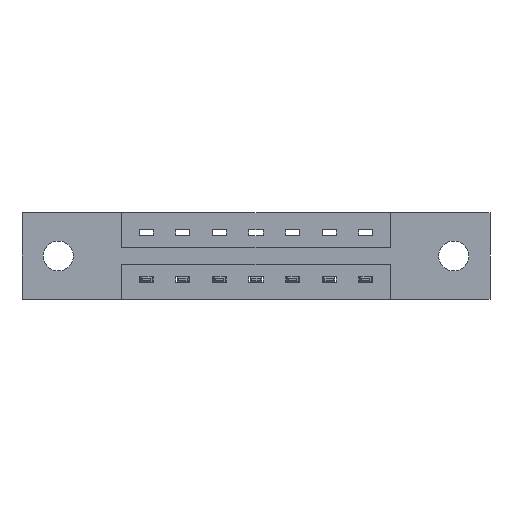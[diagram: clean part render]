
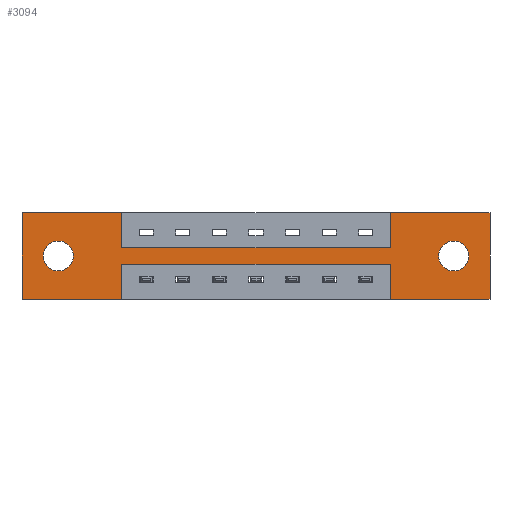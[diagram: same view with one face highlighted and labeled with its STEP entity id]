
A CAD part, front view. The second image highlights one B-rep face of the part: STEP entity #3094.
In plain terms, the highlighted planar face has unit normal (0, -1, 0).
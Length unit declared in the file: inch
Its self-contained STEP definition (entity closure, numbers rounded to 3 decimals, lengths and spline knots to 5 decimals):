
#146 = ORIENTED_EDGE ( 'NONE', *, *, #5167, .F. ) ;
#184 = ORIENTED_EDGE ( 'NONE', *, *, #8769, .F. ) ;
#269 = AXIS2_PLACEMENT_3D ( 'NONE', #9142, #9176, #1065 ) ;
#273 = VERTEX_POINT ( 'NONE', #4637 ) ;
#286 = CARTESIAN_POINT ( 'NONE',  ( 1.573, 0., -0.15 ) ) ;
#356 = CARTESIAN_POINT ( 'NONE',  ( 0.155, 0., -0.185 ) ) ;
#385 = LINE ( 'NONE', #4466, #8258 ) ;
#437 = CARTESIAN_POINT ( 'NONE',  ( 1.573, 0., -0.37 ) ) ;
#475 = VERTEX_POINT ( 'NONE', #6405 ) ;
#481 = ORIENTED_EDGE ( 'NONE', *, *, #5560, .F. ) ;
#738 = ORIENTED_EDGE ( 'NONE', *, *, #7618, .T. ) ;
#752 = LINE ( 'NONE', #7624, #9543 ) ;
#995 = DIRECTION ( 'NONE',  ( 0., 1., 0. ) ) ;
#1040 = VERTEX_POINT ( 'NONE', #6123 ) ;
#1065 = DIRECTION ( 'NONE',  ( 0., 0., 1. ) ) ;
#1081 = VERTEX_POINT ( 'NONE', #5333 ) ;
#1261 = CARTESIAN_POINT ( 'NONE',  ( 1.843, 0., -0.249 ) ) ;
#1365 = ORIENTED_EDGE ( 'NONE', *, *, #4331, .F. ) ;
#1369 = VECTOR ( 'NONE', #3549, 39.37008 ) ;
#1526 = EDGE_CURVE ( 'NONE', #7227, #5481, #5868, .T. ) ;
#1628 = LINE ( 'NONE', #2839, #7551 ) ;
#1788 = VECTOR ( 'NONE', #3250, 39.37008 ) ;
#1812 = EDGE_LOOP ( 'NONE', ( #8796, #6892 ) ) ;
#1844 = PLANE ( 'NONE',  #8091 ) ;
#1984 = VECTOR ( 'NONE', #8670, 39.37008 ) ;
#2133 = CARTESIAN_POINT ( 'NONE',  ( 1.573, 0., 0. ) ) ;
#2176 = DIRECTION ( 'NONE',  ( 0., -1., 0. ) ) ;
#2179 = CARTESIAN_POINT ( 'NONE',  ( 1.843, 0., -0.121 ) ) ;
#2238 = AXIS2_PLACEMENT_3D ( 'NONE', #7287, #5685, #8671 ) ;
#2365 = VECTOR ( 'NONE', #7357, 39.37008 ) ;
#2410 = FACE_OUTER_BOUND ( 'NONE', #8973, .T. ) ;
#2446 = CARTESIAN_POINT ( 'NONE',  ( 0., 0., 0. ) ) ;
#2516 = VERTEX_POINT ( 'NONE', #6598 ) ;
#2552 = CARTESIAN_POINT ( 'NONE',  ( 0.425, 0., -0.22 ) ) ;
#2693 = VERTEX_POINT ( 'NONE', #7929 ) ;
#2839 = CARTESIAN_POINT ( 'NONE',  ( 0., 0., 0. ) ) ;
#2935 = DIRECTION ( 'NONE',  ( 0., 1., 0. ) ) ;
#2989 = LINE ( 'NONE', #7488, #6375 ) ;
#3094 = ADVANCED_FACE ( 'NONE', ( #5359, #3254, #2410 ), #1844, .T. ) ;
#3185 = DIRECTION ( 'NONE',  ( 1., 0., 0. ) ) ;
#3238 = EDGE_CURVE ( 'NONE', #1040, #9308, #6171, .T. ) ;
#3244 = VECTOR ( 'NONE', #8270, 39.37008 ) ;
#3250 = DIRECTION ( 'NONE',  ( 0., 0., -1. ) ) ;
#3254 = FACE_BOUND ( 'NONE', #8742, .T. ) ;
#3454 = EDGE_CURVE ( 'NONE', #475, #7300, #9346, .T. ) ;
#3483 = DIRECTION ( 'NONE',  ( 0., 0., 1. ) ) ;
#3510 = EDGE_CURVE ( 'NONE', #6301, #4261, #7523, .T. ) ;
#3518 = DIRECTION ( 'NONE',  ( 0., 0., 1. ) ) ;
#3549 = DIRECTION ( 'NONE',  ( 1., 0., 0. ) ) ;
#3720 = VECTOR ( 'NONE', #8417, 39.37008 ) ;
#3864 = EDGE_CURVE ( 'NONE', #2693, #4947, #8649, .T. ) ;
#3933 = VECTOR ( 'NONE', #3185, 39.37008 ) ;
#4011 = ORIENTED_EDGE ( 'NONE', *, *, #5133, .F. ) ;
#4071 = CARTESIAN_POINT ( 'NONE',  ( 0.425, 0., 0. ) ) ;
#4094 = ORIENTED_EDGE ( 'NONE', *, *, #8106, .F. ) ;
#4213 = EDGE_CURVE ( 'NONE', #6529, #8342, #2989, .T. ) ;
#4261 = VERTEX_POINT ( 'NONE', #4685 ) ;
#4331 = EDGE_CURVE ( 'NONE', #8342, #2693, #752, .T. ) ;
#4466 = CARTESIAN_POINT ( 'NONE',  ( 0.425, 0., 0. ) ) ;
#4637 = CARTESIAN_POINT ( 'NONE',  ( 1.998, 0., 0. ) ) ;
#4673 = LINE ( 'NONE', #2552, #3720 ) ;
#4682 = CARTESIAN_POINT ( 'NONE',  ( 1.573, 0., 0. ) ) ;
#4685 = CARTESIAN_POINT ( 'NONE',  ( 1.573, 0., -0.37 ) ) ;
#4721 = CARTESIAN_POINT ( 'NONE',  ( 0.425, 0., -0.37 ) ) ;
#4798 = ORIENTED_EDGE ( 'NONE', *, *, #3510, .F. ) ;
#4842 = DIRECTION ( 'NONE',  ( 0., 0., 1. ) ) ;
#4947 = VERTEX_POINT ( 'NONE', #4071 ) ;
#4964 = CARTESIAN_POINT ( 'NONE',  ( 1.998, 0., 0. ) ) ;
#5046 = LINE ( 'NONE', #437, #5992 ) ;
#5067 = DIRECTION ( 'NONE',  ( 1., 0., 0. ) ) ;
#5133 = EDGE_CURVE ( 'NONE', #1081, #6529, #5783, .T. ) ;
#5161 = CIRCLE ( 'NONE', #5441, 0.064 ) ;
#5167 = EDGE_CURVE ( 'NONE', #9308, #7965, #9062, .T. ) ;
#5232 = DIRECTION ( 'NONE',  ( -1., 0., 0. ) ) ;
#5333 = CARTESIAN_POINT ( 'NONE',  ( 0.425, 0., -0.22 ) ) ;
#5359 = FACE_BOUND ( 'NONE', #1812, .T. ) ;
#5441 = AXIS2_PLACEMENT_3D ( 'NONE', #356, #995, #4842 ) ;
#5481 = VERTEX_POINT ( 'NONE', #2179 ) ;
#5525 = ORIENTED_EDGE ( 'NONE', *, *, #6911, .F. ) ;
#5560 = EDGE_CURVE ( 'NONE', #4947, #1040, #385, .T. ) ;
#5685 = DIRECTION ( 'NONE',  ( 0., 1., 0. ) ) ;
#5783 = LINE ( 'NONE', #4721, #1788 ) ;
#5863 = CARTESIAN_POINT ( 'NONE',  ( 1.843, 0., -0.185 ) ) ;
#5868 = CIRCLE ( 'NONE', #2238, 0.064 ) ;
#5900 = CARTESIAN_POINT ( 'NONE',  ( 0.155, 0., -0.121 ) ) ;
#5915 = EDGE_CURVE ( 'NONE', #5481, #7227, #8938, .T. ) ;
#5992 = VECTOR ( 'NONE', #3518, 39.37008 ) ;
#6123 = CARTESIAN_POINT ( 'NONE',  ( 0.425, 0., -0.15 ) ) ;
#6171 = LINE ( 'NONE', #7204, #1369 ) ;
#6176 = EDGE_CURVE ( 'NONE', #273, #6301, #9280, .T. ) ;
#6225 = CARTESIAN_POINT ( 'NONE',  ( 0., 0., -0.37 ) ) ;
#6301 = VERTEX_POINT ( 'NONE', #6687 ) ;
#6355 = CARTESIAN_POINT ( 'NONE',  ( 0., 0., -0.37 ) ) ;
#6375 = VECTOR ( 'NONE', #5232, 39.37008 ) ;
#6405 = CARTESIAN_POINT ( 'NONE',  ( 0.155, 0., -0.249 ) ) ;
#6458 = CARTESIAN_POINT ( 'NONE',  ( 0.425, 0., -0.37 ) ) ;
#6529 = VERTEX_POINT ( 'NONE', #6458 ) ;
#6587 = DIRECTION ( 'NONE',  ( 0., 0., -1. ) ) ;
#6598 = CARTESIAN_POINT ( 'NONE',  ( 1.573, 0., -0.22 ) ) ;
#6609 = CARTESIAN_POINT ( 'NONE',  ( 0., 0., -0.37 ) ) ;
#6687 = CARTESIAN_POINT ( 'NONE',  ( 1.998, 0., -0.37 ) ) ;
#6835 = DIRECTION ( 'NONE',  ( 0., 0., -1. ) ) ;
#6892 = ORIENTED_EDGE ( 'NONE', *, *, #1526, .T. ) ;
#6911 = EDGE_CURVE ( 'NONE', #4261, #2516, #5046, .T. ) ;
#7204 = CARTESIAN_POINT ( 'NONE',  ( 0.425, 0., -0.15 ) ) ;
#7227 = VERTEX_POINT ( 'NONE', #1261 ) ;
#7287 = CARTESIAN_POINT ( 'NONE',  ( 1.843, 0., -0.185 ) ) ;
#7300 = VERTEX_POINT ( 'NONE', #5900 ) ;
#7357 = DIRECTION ( 'NONE',  ( 0., 0., 1. ) ) ;
#7368 = ORIENTED_EDGE ( 'NONE', *, *, #3454, .T. ) ;
#7488 = CARTESIAN_POINT ( 'NONE',  ( 0., 0., -0.37 ) ) ;
#7523 = LINE ( 'NONE', #6225, #3244 ) ;
#7551 = VECTOR ( 'NONE', #5067, 39.37008 ) ;
#7618 = EDGE_CURVE ( 'NONE', #7300, #475, #5161, .T. ) ;
#7624 = CARTESIAN_POINT ( 'NONE',  ( 0., 0., 0. ) ) ;
#7845 = ORIENTED_EDGE ( 'NONE', *, *, #3238, .F. ) ;
#7929 = CARTESIAN_POINT ( 'NONE',  ( 0., 0., 0. ) ) ;
#7965 = VERTEX_POINT ( 'NONE', #4682 ) ;
#8091 = AXIS2_PLACEMENT_3D ( 'NONE', #6355, #2176, #8284 ) ;
#8106 = EDGE_CURVE ( 'NONE', #7965, #273, #1628, .T. ) ;
#8258 = VECTOR ( 'NONE', #6835, 39.37008 ) ;
#8270 = DIRECTION ( 'NONE',  ( -1., 0., 0. ) ) ;
#8284 = DIRECTION ( 'NONE',  ( 0., 0., -1. ) ) ;
#8342 = VERTEX_POINT ( 'NONE', #6609 ) ;
#8417 = DIRECTION ( 'NONE',  ( -1., 0., 0. ) ) ;
#8528 = ORIENTED_EDGE ( 'NONE', *, *, #4213, .F. ) ;
#8649 = LINE ( 'NONE', #2446, #3933 ) ;
#8670 = DIRECTION ( 'NONE',  ( 0., 0., -1. ) ) ;
#8671 = DIRECTION ( 'NONE',  ( 0., 0., -1. ) ) ;
#8742 = EDGE_LOOP ( 'NONE', ( #738, #7368 ) ) ;
#8769 = EDGE_CURVE ( 'NONE', #2516, #1081, #4673, .T. ) ;
#8796 = ORIENTED_EDGE ( 'NONE', *, *, #5915, .T. ) ;
#8938 = CIRCLE ( 'NONE', #9520, 0.064 ) ;
#8973 = EDGE_LOOP ( 'NONE', ( #4011, #184, #5525, #4798, #9082, #4094, #146, #7845, #481, #9553, #1365, #8528 ) ) ;
#9062 = LINE ( 'NONE', #2133, #2365 ) ;
#9082 = ORIENTED_EDGE ( 'NONE', *, *, #6176, .F. ) ;
#9142 = CARTESIAN_POINT ( 'NONE',  ( 0.155, 0., -0.185 ) ) ;
#9176 = DIRECTION ( 'NONE',  ( 0., 1., 0. ) ) ;
#9280 = LINE ( 'NONE', #4964, #1984 ) ;
#9308 = VERTEX_POINT ( 'NONE', #286 ) ;
#9346 = CIRCLE ( 'NONE', #269, 0.064 ) ;
#9520 = AXIS2_PLACEMENT_3D ( 'NONE', #5863, #2935, #6587 ) ;
#9543 = VECTOR ( 'NONE', #3483, 39.37008 ) ;
#9553 = ORIENTED_EDGE ( 'NONE', *, *, #3864, .F. ) ;
